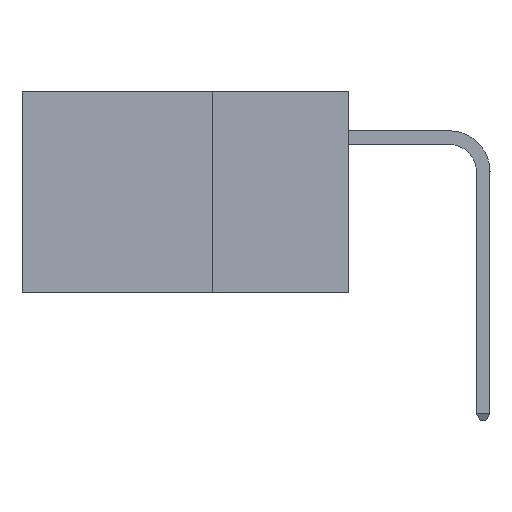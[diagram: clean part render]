
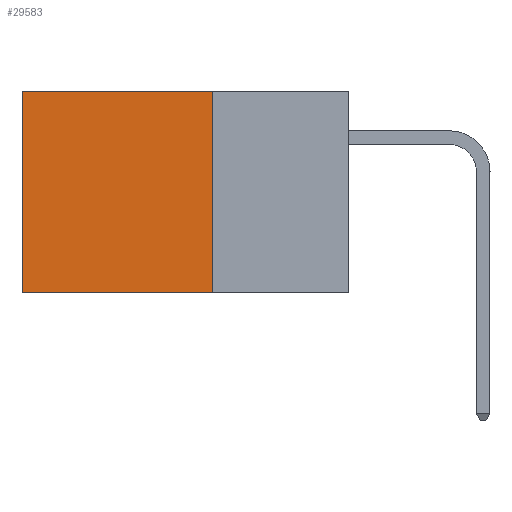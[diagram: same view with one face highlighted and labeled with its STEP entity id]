
A CAD part, left-side view. The second image highlights one B-rep face of the part: STEP entity #29583.
In plain terms, the highlighted planar face has unit normal (-1, 0, 0).
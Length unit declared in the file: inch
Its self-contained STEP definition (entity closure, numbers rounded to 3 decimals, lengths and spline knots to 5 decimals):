
#1294 = LINE ( 'NONE', #37609, #38896 ) ;
#2517 = DIRECTION ( 'NONE',  ( 0., 0., -1. ) ) ;
#2579 = CARTESIAN_POINT ( 'NONE',  ( 0.2875, 0.25, 0. ) ) ;
#7336 = CARTESIAN_POINT ( 'NONE',  ( 0.2875, 0.6, 0. ) ) ;
#13941 = EDGE_CURVE ( 'NONE', #35373, #17385, #1294, .T. ) ;
#14813 = ORIENTED_EDGE ( 'NONE', *, *, #32575, .T. ) ;
#17385 = VERTEX_POINT ( 'NONE', #27154 ) ;
#18166 = PLANE ( 'NONE',  #29663 ) ;
#19728 = LINE ( 'NONE', #28544, #49456 ) ;
#25335 = DIRECTION ( 'NONE',  ( 1., 0., 0. ) ) ;
#25507 = CARTESIAN_POINT ( 'NONE',  ( 0.2875, 0.25, 0. ) ) ;
#26729 = CARTESIAN_POINT ( 'NONE',  ( 0.2875, 0.25, 0. ) ) ;
#27154 = CARTESIAN_POINT ( 'NONE',  ( 0.2875, 0.25, -0.37 ) ) ;
#27812 = LINE ( 'NONE', #2579, #45997 ) ;
#28544 = CARTESIAN_POINT ( 'NONE',  ( 0.2875, 0.25, -0.37 ) ) ;
#29583 = ADVANCED_FACE ( 'NONE', ( #34625 ), #18166, .F. ) ;
#29663 = AXIS2_PLACEMENT_3D ( 'NONE', #25507, #25335, #45334 ) ;
#30332 = ORIENTED_EDGE ( 'NONE', *, *, #45707, .F. ) ;
#32575 = EDGE_CURVE ( 'NONE', #35008, #40156, #48198, .T. ) ;
#34625 = FACE_OUTER_BOUND ( 'NONE', #40745, .T. ) ;
#35008 = VERTEX_POINT ( 'NONE', #43009 ) ;
#35373 = VERTEX_POINT ( 'NONE', #26729 ) ;
#37609 = CARTESIAN_POINT ( 'NONE',  ( 0.2875, 0.25, 0. ) ) ;
#38051 = ORIENTED_EDGE ( 'NONE', *, *, #13941, .F. ) ;
#38896 = VECTOR ( 'NONE', #2517, 39.37008 ) ;
#40056 = DIRECTION ( 'NONE',  ( 0., 1., 0. ) ) ;
#40156 = VERTEX_POINT ( 'NONE', #46561 ) ;
#40524 = EDGE_CURVE ( 'NONE', #35373, #35008, #27812, .T. ) ;
#40745 = EDGE_LOOP ( 'NONE', ( #14813, #30332, #38051, #50199 ) ) ;
#43009 = CARTESIAN_POINT ( 'NONE',  ( 0.2875, 0.6, 0. ) ) ;
#45334 = DIRECTION ( 'NONE',  ( 0., 0., -1. ) ) ;
#45707 = EDGE_CURVE ( 'NONE', #17385, #40156, #19728, .T. ) ;
#45786 = VECTOR ( 'NONE', #46168, 39.37008 ) ;
#45997 = VECTOR ( 'NONE', #49528, 39.37008 ) ;
#46168 = DIRECTION ( 'NONE',  ( 0., 0., -1. ) ) ;
#46561 = CARTESIAN_POINT ( 'NONE',  ( 0.2875, 0.6, -0.37 ) ) ;
#48198 = LINE ( 'NONE', #7336, #45786 ) ;
#49456 = VECTOR ( 'NONE', #40056, 39.37008 ) ;
#49528 = DIRECTION ( 'NONE',  ( 0., 1., 0. ) ) ;
#50199 = ORIENTED_EDGE ( 'NONE', *, *, #40524, .T. ) ;
